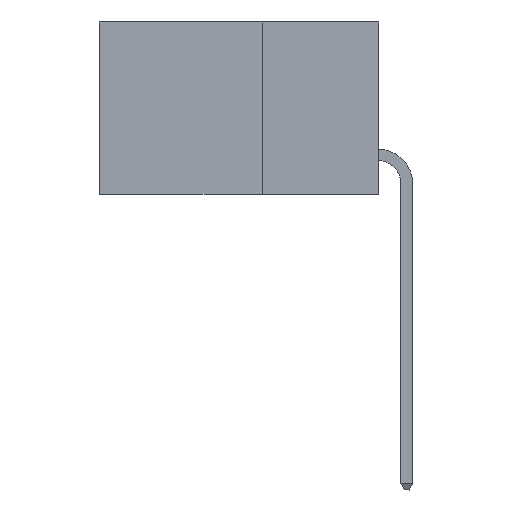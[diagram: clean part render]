
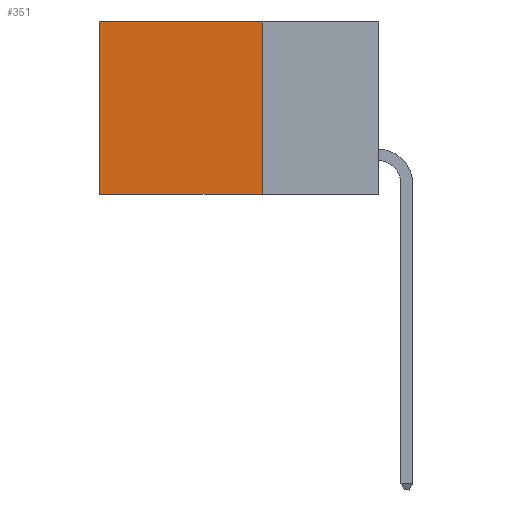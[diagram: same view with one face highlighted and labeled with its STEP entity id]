
A CAD part, left-side view. The second image highlights one B-rep face of the part: STEP entity #351.
In plain terms, the highlighted planar face has unit normal (-1, 0, 0).
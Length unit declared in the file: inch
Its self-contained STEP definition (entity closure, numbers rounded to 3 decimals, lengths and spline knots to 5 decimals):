
#351 = ADVANCED_FACE ( 'NONE', ( #4703 ), #8173, .F. ) ;
#523 = CARTESIAN_POINT ( 'NONE',  ( 0.2615, 0.6, -0.37 ) ) ;
#1040 = VERTEX_POINT ( 'NONE', #8849 ) ;
#1128 = EDGE_CURVE ( 'NONE', #11125, #8454, #8029, .T. ) ;
#1260 = EDGE_CURVE ( 'NONE', #1300, #11125, #10911, .T. ) ;
#1300 = VERTEX_POINT ( 'NONE', #4668 ) ;
#1640 = CARTESIAN_POINT ( 'NONE',  ( 0.2615, 0.25, -0.37 ) ) ;
#1722 = CARTESIAN_POINT ( 'NONE',  ( 0.2615, 0.25, 0. ) ) ;
#2130 = AXIS2_PLACEMENT_3D ( 'NONE', #3812, #3641, #2681 ) ;
#2135 = CARTESIAN_POINT ( 'NONE',  ( 0.2615, 0.6, -0.37 ) ) ;
#2442 = ORIENTED_EDGE ( 'NONE', *, *, #1128, .F. ) ;
#2681 = DIRECTION ( 'NONE',  ( 0., 0., -1. ) ) ;
#3501 = VECTOR ( 'NONE', #4235, 39.37008 ) ;
#3641 = DIRECTION ( 'NONE',  ( 1., 0., 0. ) ) ;
#3812 = CARTESIAN_POINT ( 'NONE',  ( 0.2615, 0.25, -0.37 ) ) ;
#3988 = VECTOR ( 'NONE', #8366, 39.37008 ) ;
#4235 = DIRECTION ( 'NONE',  ( 0., 0., -1. ) ) ;
#4261 = EDGE_CURVE ( 'NONE', #1040, #8454, #11549, .T. ) ;
#4668 = CARTESIAN_POINT ( 'NONE',  ( 0.2615, 0.25, 0. ) ) ;
#4703 = FACE_OUTER_BOUND ( 'NONE', #6753, .T. ) ;
#4994 = ORIENTED_EDGE ( 'NONE', *, *, #4261, .T. ) ;
#5245 = DIRECTION ( 'NONE',  ( 0., 1., 0. ) ) ;
#6161 = ORIENTED_EDGE ( 'NONE', *, *, #1260, .F. ) ;
#6213 = LINE ( 'NONE', #1722, #10535 ) ;
#6753 = EDGE_LOOP ( 'NONE', ( #4994, #2442, #6161, #7685 ) ) ;
#7363 = EDGE_CURVE ( 'NONE', #1300, #1040, #6213, .T. ) ;
#7685 = ORIENTED_EDGE ( 'NONE', *, *, #7363, .T. ) ;
#8029 = LINE ( 'NONE', #1640, #9917 ) ;
#8173 = PLANE ( 'NONE',  #2130 ) ;
#8245 = CARTESIAN_POINT ( 'NONE',  ( 0.2615, 0.25, -0.37 ) ) ;
#8366 = DIRECTION ( 'NONE',  ( 0., 0., -1. ) ) ;
#8454 = VERTEX_POINT ( 'NONE', #2135 ) ;
#8773 = CARTESIAN_POINT ( 'NONE',  ( 0.2615, 0.25, -0.37 ) ) ;
#8849 = CARTESIAN_POINT ( 'NONE',  ( 0.2615, 0.6, 0. ) ) ;
#9917 = VECTOR ( 'NONE', #11627, 39.37008 ) ;
#10535 = VECTOR ( 'NONE', #5245, 39.37008 ) ;
#10911 = LINE ( 'NONE', #8245, #3988 ) ;
#11125 = VERTEX_POINT ( 'NONE', #8773 ) ;
#11549 = LINE ( 'NONE', #523, #3501 ) ;
#11627 = DIRECTION ( 'NONE',  ( 0., 1., 0. ) ) ;
